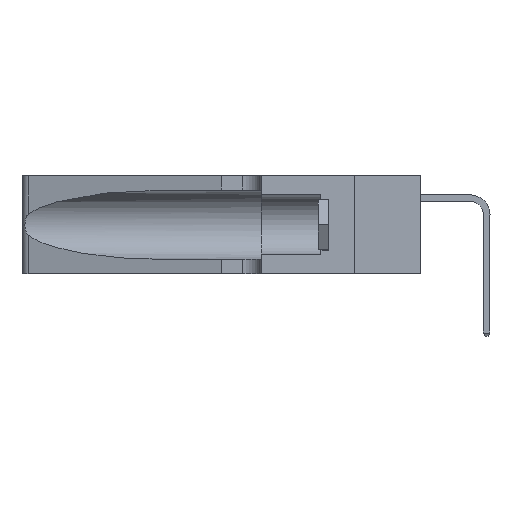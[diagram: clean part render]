
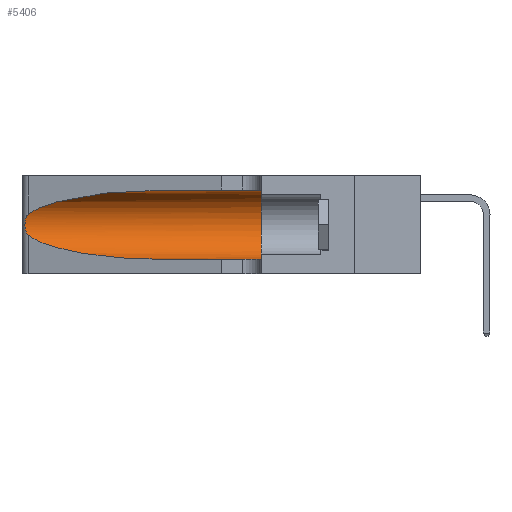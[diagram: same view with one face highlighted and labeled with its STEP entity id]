
A CAD part, left-side view. The second image highlights one B-rep face of the part: STEP entity #5406.
In plain terms, the highlighted cylindrical face has radius 3.308 mm (diameter 6.617 mm), a partial arc.
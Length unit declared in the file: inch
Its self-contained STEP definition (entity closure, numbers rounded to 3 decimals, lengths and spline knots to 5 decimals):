
#589 = ORIENTED_EDGE ( 'NONE', *, *, #6319, .T. ) ;
#845 = CARTESIAN_POINT ( 'NONE',  ( 0.26018, 1.23835, 0.19895 ) ) ;
#1058 = DIRECTION ( 'NONE',  ( 0., -1., 0. ) ) ;
#1090 = CARTESIAN_POINT ( 'NONE',  ( 0.2373, 1.15595, 0.08982 ) ) ;
#1360 = EDGE_CURVE ( 'NONE', #21859, #15233, #17020, .T. ) ;
#1412 = EDGE_LOOP ( 'NONE', ( #11810, #2099, #5161, #589, #17858, #5238 ) ) ;
#2042 = LINE ( 'NONE', #10485, #10826 ) ;
#2099 = ORIENTED_EDGE ( 'NONE', *, *, #17157, .T. ) ;
#2198 = VERTEX_POINT ( 'NONE', #8210 ) ;
#2630 = CARTESIAN_POINT ( 'NONE',  ( 0.26075, 1.23896, 0.178 ) ) ;
#3994 = VERTEX_POINT ( 'NONE', #17288 ) ;
#4225 = CIRCLE ( 'NONE', #11801, 0.13025 ) ;
#4410 = CARTESIAN_POINT ( 'NONE',  ( 0.25856, 1.23593, 0.16098 ) ) ;
#4932 = CARTESIAN_POINT ( 'NONE',  ( 0.1305, 0.35, 0.185 ) ) ;
#5161 = ORIENTED_EDGE ( 'NONE', *, *, #18613, .T. ) ;
#5238 = ORIENTED_EDGE ( 'NONE', *, *, #18167, .F. ) ;
#5406 = ADVANCED_FACE ( 'NONE', ( #21665 ), #7652, .F. ) ;
#5581 = AXIS2_PLACEMENT_3D ( 'NONE', #22743, #12263, #19227 ) ;
#6089 = CARTESIAN_POINT ( 'NONE',  ( 0.25555, 1.22994, 0.2215 ) ) ;
#6161 = CARTESIAN_POINT ( 'NONE',  ( 0.25639, 1.23186, 0.15144 ) ) ;
#6319 = EDGE_CURVE ( 'NONE', #3994, #13966, #10641, .T. ) ;
#6409 = CARTESIAN_POINT ( 'NONE',  ( 0.25487, 1.22718, 0.14631 ) ) ;
#6681 = DIRECTION ( 'NONE',  ( 0., 0., 1. ) ) ;
#7652 = CYLINDRICAL_SURFACE ( 'NONE', #5581, 0.13025 ) ;
#7838 = CARTESIAN_POINT ( 'NONE',  ( 0.25487, 1.22718, 0.22369 ) ) ;
#7929 = CARTESIAN_POINT ( 'NONE',  ( 0.25487, 1.22718, 0.14631 ) ) ;
#8210 = CARTESIAN_POINT ( 'NONE',  ( 0.25487, 1.22718, 0.14631 ) ) ;
#9314 = CARTESIAN_POINT ( 'NONE',  ( 0.1305, 0.72297, 0.31525 ) ) ;
#9381 = CARTESIAN_POINT ( 'NONE',  ( 0.18966, 0.96281, 0.31525 ) ) ;
#9610 = CARTESIAN_POINT ( 'NONE',  ( 0.25639, 1.23184, 0.21858 ) ) ;
#10485 = CARTESIAN_POINT ( 'NONE',  ( 0.1305, 1.61858, 0.31525 ) ) ;
#10641 = LINE ( 'NONE', #18568, #14764 ) ;
#10731 = CARTESIAN_POINT ( 'NONE',  ( 0.1305, 0.35, 0.05475 ) ) ;
#10826 = VECTOR ( 'NONE', #13949, 39.37008 ) ;
#11159 = CARTESIAN_POINT ( 'NONE',  ( 0.25487, 1.22718, 0.22369 ) ) ;
#11386 = CARTESIAN_POINT ( 'NONE',  ( 0.25854, 1.2359, 0.20912 ) ) ;
#11716 = CARTESIAN_POINT ( 'NONE',  ( 0.1305, 0.72297, 0.05475 ) ) ;
#11801 = AXIS2_PLACEMENT_3D ( 'NONE', #4932, #17186, #6681 ) ;
#11810 = ORIENTED_EDGE ( 'NONE', *, *, #1360, .T. ) ;
#12263 = DIRECTION ( 'NONE',  ( 0., -1., 0. ) ) ;
#13145 = CARTESIAN_POINT ( 'NONE',  ( 0.26075, 1.23896, 0.19203 ) ) ;
#13949 = DIRECTION ( 'NONE',  ( 0., -1., 0. ) ) ;
#13966 = VERTEX_POINT ( 'NONE', #10731 ) ;
#14411 =( BOUNDED_CURVE ( )  B_SPLINE_CURVE ( 3, ( #6409, #1090, #22204, #11716 ),
 .UNSPECIFIED., .F., .T. ) 
 B_SPLINE_CURVE_WITH_KNOTS ( ( 4, 4 ),
 ( 3.44316, 4.71239 ),
 .UNSPECIFIED. ) 
 CURVE ( )  GEOMETRIC_REPRESENTATION_ITEM ( )  RATIONAL_B_SPLINE_CURVE ( ( 1., 0.87, 0.87, 1. ) ) 
 REPRESENTATION_ITEM ( '' )  );
#14599 = CARTESIAN_POINT ( 'NONE',  ( 0.25487, 1.22718, 0.22369 ) ) ;
#14764 = VECTOR ( 'NONE', #1058, 39.37008 ) ;
#14906 = CARTESIAN_POINT ( 'NONE',  ( 0.26017, 1.23833, 0.17102 ) ) ;
#15041 = B_SPLINE_CURVE_WITH_KNOTS ( 'NONE', 3,
 ( #7838, #6089, #9610, #21886, #11386, #845, #13145, #2630, #14906, #4410, #16650, #6161, #18435, #7929 ),
 .UNSPECIFIED., .F., .F.,
 ( 4, 2, 2, 2, 2, 2, 4 ),
 ( 0., 0.00027, 0.00053, 0.00107, 0.0016, 0.00187, 0.00214 ),
 .UNSPECIFIED. ) ;
#15233 = VERTEX_POINT ( 'NONE', #14599 ) ;
#16650 = CARTESIAN_POINT ( 'NONE',  ( 0.25789, 1.23486, 0.15765 ) ) ;
#17020 =( BOUNDED_CURVE ( )  B_SPLINE_CURVE ( 3, ( #9314, #9381, #19875, #11159 ),
 .UNSPECIFIED., .F., .F. ) 
 B_SPLINE_CURVE_WITH_KNOTS ( ( 4, 4 ),
 ( 1.5708, 2.84003 ),
 .UNSPECIFIED. ) 
 CURVE ( )  GEOMETRIC_REPRESENTATION_ITEM ( )  RATIONAL_B_SPLINE_CURVE ( ( 1., 0.87, 0.87, 1. ) ) 
 REPRESENTATION_ITEM ( '' )  );
#17157 = EDGE_CURVE ( 'NONE', #15233, #2198, #15041, .T. ) ;
#17186 = DIRECTION ( 'NONE',  ( 0., 1., 0. ) ) ;
#17288 = CARTESIAN_POINT ( 'NONE',  ( 0.1305, 0.72297, 0.05475 ) ) ;
#17307 = CARTESIAN_POINT ( 'NONE',  ( 0.1305, 0.72297, 0.31525 ) ) ;
#17858 = ORIENTED_EDGE ( 'NONE', *, *, #19314, .F. ) ;
#18167 = EDGE_CURVE ( 'NONE', #21859, #21159, #2042, .T. ) ;
#18435 = CARTESIAN_POINT ( 'NONE',  ( 0.25555, 1.22993, 0.14849 ) ) ;
#18568 = CARTESIAN_POINT ( 'NONE',  ( 0.1305, 1.61858, 0.05475 ) ) ;
#18613 = EDGE_CURVE ( 'NONE', #2198, #3994, #14411, .T. ) ;
#19227 = DIRECTION ( 'NONE',  ( 0., 0., -1. ) ) ;
#19314 = EDGE_CURVE ( 'NONE', #21159, #13966, #4225, .T. ) ;
#19875 = CARTESIAN_POINT ( 'NONE',  ( 0.2373, 1.15595, 0.28018 ) ) ;
#21159 = VERTEX_POINT ( 'NONE', #22085 ) ;
#21665 = FACE_OUTER_BOUND ( 'NONE', #1412, .T. ) ;
#21859 = VERTEX_POINT ( 'NONE', #17307 ) ;
#21886 = CARTESIAN_POINT ( 'NONE',  ( 0.25787, 1.23484, 0.2124 ) ) ;
#22085 = CARTESIAN_POINT ( 'NONE',  ( 0.1305, 0.35, 0.31525 ) ) ;
#22204 = CARTESIAN_POINT ( 'NONE',  ( 0.18966, 0.96281, 0.05475 ) ) ;
#22743 = CARTESIAN_POINT ( 'NONE',  ( 0.1305, 1.61858, 0.185 ) ) ;
